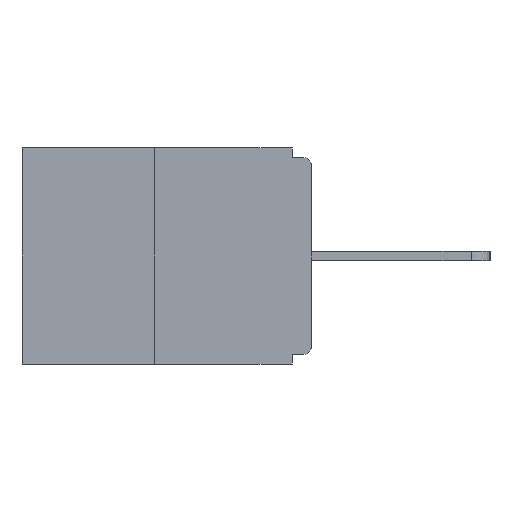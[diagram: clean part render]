
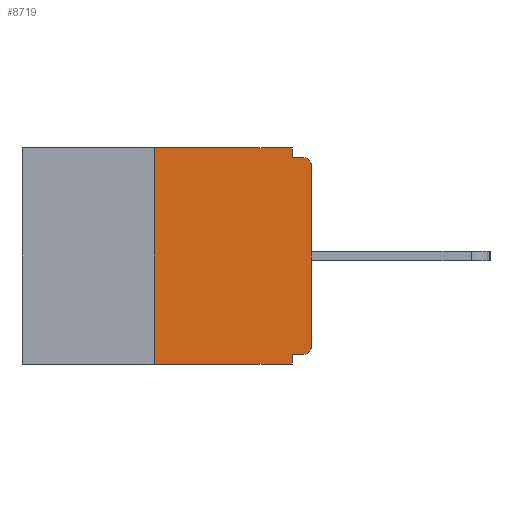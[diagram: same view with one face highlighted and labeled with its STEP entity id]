
A CAD part, left-side view. The second image highlights one B-rep face of the part: STEP entity #8719.
In plain terms, the highlighted planar face has unit normal (-1, 0, 0).
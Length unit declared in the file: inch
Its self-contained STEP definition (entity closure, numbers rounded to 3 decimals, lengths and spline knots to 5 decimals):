
#188 = CARTESIAN_POINT ( 'NONE',  ( 0., 0.031, 0. ) ) ;
#361 = ORIENTED_EDGE ( 'NONE', *, *, #2135, .F. ) ;
#524 = LINE ( 'NONE', #4697, #8600 ) ;
#560 = CARTESIAN_POINT ( 'NONE',  ( 0., 0.25, 0. ) ) ;
#567 = ORIENTED_EDGE ( 'NONE', *, *, #5342, .F. ) ;
#771 = DIRECTION ( 'NONE',  ( 1., 0., 0. ) ) ;
#990 = DIRECTION ( 'NONE',  ( 0., 0., -1. ) ) ;
#1240 = LINE ( 'NONE', #10853, #4641 ) ;
#1313 = CARTESIAN_POINT ( 'NONE',  ( 0., 0., -0.328 ) ) ;
#1405 = AXIS2_PLACEMENT_3D ( 'NONE', #8255, #771, #9372 ) ;
#1598 = CIRCLE ( 'NONE', #12815, 0.015 ) ;
#1734 = EDGE_LOOP ( 'NONE', ( #7127, #5893, #7165, #567, #10766, #7351, #2995, #6404, #7505, #361 ) ) ;
#1804 = DIRECTION ( 'NONE',  ( 0., -1., 0. ) ) ;
#1980 = CARTESIAN_POINT ( 'NONE',  ( 0., 0.015, -0.015 ) ) ;
#2005 = FACE_OUTER_BOUND ( 'NONE', #1734, .T. ) ;
#2135 = EDGE_CURVE ( 'NONE', #13423, #8696, #4157, .T. ) ;
#2299 = VECTOR ( 'NONE', #1804, 39.37008 ) ;
#2954 = CARTESIAN_POINT ( 'NONE',  ( 0., 0.031, -0.328 ) ) ;
#2995 = ORIENTED_EDGE ( 'NONE', *, *, #7608, .T. ) ;
#3349 = VERTEX_POINT ( 'NONE', #7394 ) ;
#3566 = DIRECTION ( 'NONE',  ( 0., 1., 0. ) ) ;
#3804 = VECTOR ( 'NONE', #9778, 39.37008 ) ;
#3986 = CARTESIAN_POINT ( 'NONE',  ( 0., 0., -0.015 ) ) ;
#4157 = LINE ( 'NONE', #188, #4753 ) ;
#4296 = DIRECTION ( 'NONE',  ( 0., 0., 1. ) ) ;
#4641 = VECTOR ( 'NONE', #4296, 39.37008 ) ;
#4697 = CARTESIAN_POINT ( 'NONE',  ( 0., 0.46, -0.343 ) ) ;
#4753 = VECTOR ( 'NONE', #5257, 39.37008 ) ;
#4831 = CARTESIAN_POINT ( 'NONE',  ( 0., 0.031, 0. ) ) ;
#5257 = DIRECTION ( 'NONE',  ( 0., 0., -1. ) ) ;
#5342 = EDGE_CURVE ( 'NONE', #7071, #12748, #8388, .T. ) ;
#5519 = EDGE_CURVE ( 'NONE', #10496, #13423, #8584, .T. ) ;
#5863 = VERTEX_POINT ( 'NONE', #7185 ) ;
#5893 = ORIENTED_EDGE ( 'NONE', *, *, #10314, .F. ) ;
#6404 = ORIENTED_EDGE ( 'NONE', *, *, #6942, .T. ) ;
#6863 = LINE ( 'NONE', #1313, #9118 ) ;
#6876 = DIRECTION ( 'NONE',  ( 0., 0., -1. ) ) ;
#6942 = EDGE_CURVE ( 'NONE', #3349, #12597, #1598, .T. ) ;
#7071 = VERTEX_POINT ( 'NONE', #2954 ) ;
#7127 = ORIENTED_EDGE ( 'NONE', *, *, #5519, .F. ) ;
#7131 = CARTESIAN_POINT ( 'NONE',  ( 0., 0.25, 0. ) ) ;
#7165 = ORIENTED_EDGE ( 'NONE', *, *, #7809, .T. ) ;
#7185 = CARTESIAN_POINT ( 'NONE',  ( 0., 0.015, -0.328 ) ) ;
#7351 = ORIENTED_EDGE ( 'NONE', *, *, #13072, .T. ) ;
#7394 = CARTESIAN_POINT ( 'NONE',  ( 0., 0., -0.03 ) ) ;
#7416 = VERTEX_POINT ( 'NONE', #13518 ) ;
#7505 = ORIENTED_EDGE ( 'NONE', *, *, #13149, .F. ) ;
#7608 = EDGE_CURVE ( 'NONE', #11166, #3349, #1240, .T. ) ;
#7755 = AXIS2_PLACEMENT_3D ( 'NONE', #8949, #9095, #6876 ) ;
#7809 = EDGE_CURVE ( 'NONE', #7416, #12748, #524, .T. ) ;
#8102 = PLANE ( 'NONE',  #1405 ) ;
#8255 = CARTESIAN_POINT ( 'NONE',  ( 0., 0.46, 0. ) ) ;
#8388 = LINE ( 'NONE', #10546, #11446 ) ;
#8560 = CARTESIAN_POINT ( 'NONE',  ( 0., 0., -0.313 ) ) ;
#8584 = LINE ( 'NONE', #12832, #9665 ) ;
#8600 = VECTOR ( 'NONE', #8921, 39.37008 ) ;
#8696 = VERTEX_POINT ( 'NONE', #13598 ) ;
#8719 = ADVANCED_FACE ( 'NONE', ( #2005 ), #8102, .F. ) ;
#8921 = DIRECTION ( 'NONE',  ( 0., -1., 0. ) ) ;
#8949 = CARTESIAN_POINT ( 'NONE',  ( 0., 0.015, -0.313 ) ) ;
#9095 = DIRECTION ( 'NONE',  ( -1., 0., 0. ) ) ;
#9118 = VECTOR ( 'NONE', #3566, 39.37008 ) ;
#9372 = DIRECTION ( 'NONE',  ( 0., 0., -1. ) ) ;
#9665 = VECTOR ( 'NONE', #10749, 39.37008 ) ;
#9778 = DIRECTION ( 'NONE',  ( 0., 0., 1. ) ) ;
#10314 = EDGE_CURVE ( 'NONE', #7416, #10496, #12143, .T. ) ;
#10496 = VERTEX_POINT ( 'NONE', #7131 ) ;
#10546 = CARTESIAN_POINT ( 'NONE',  ( 0., 0.031, -0.343 ) ) ;
#10649 = CIRCLE ( 'NONE', #7755, 0.015 ) ;
#10719 = CARTESIAN_POINT ( 'NONE',  ( 0., 0.031, -0.343 ) ) ;
#10749 = DIRECTION ( 'NONE',  ( 0., -1., 0. ) ) ;
#10766 = ORIENTED_EDGE ( 'NONE', *, *, #12026, .F. ) ;
#10853 = CARTESIAN_POINT ( 'NONE',  ( 0., 0., 0. ) ) ;
#10906 = CARTESIAN_POINT ( 'NONE',  ( 0., 0.015, -0.03 ) ) ;
#11166 = VERTEX_POINT ( 'NONE', #8560 ) ;
#11436 = DIRECTION ( 'NONE',  ( -1., 0., 0. ) ) ;
#11446 = VECTOR ( 'NONE', #990, 39.37008 ) ;
#12026 = EDGE_CURVE ( 'NONE', #5863, #7071, #6863, .T. ) ;
#12143 = LINE ( 'NONE', #560, #3804 ) ;
#12351 = LINE ( 'NONE', #3986, #2299 ) ;
#12550 = DIRECTION ( 'NONE',  ( 0., 0., -1. ) ) ;
#12597 = VERTEX_POINT ( 'NONE', #1980 ) ;
#12748 = VERTEX_POINT ( 'NONE', #10719 ) ;
#12815 = AXIS2_PLACEMENT_3D ( 'NONE', #10906, #11436, #12550 ) ;
#12832 = CARTESIAN_POINT ( 'NONE',  ( 0., 0.46, 0. ) ) ;
#13072 = EDGE_CURVE ( 'NONE', #5863, #11166, #10649, .T. ) ;
#13149 = EDGE_CURVE ( 'NONE', #8696, #12597, #12351, .T. ) ;
#13423 = VERTEX_POINT ( 'NONE', #4831 ) ;
#13518 = CARTESIAN_POINT ( 'NONE',  ( 0., 0.25, -0.343 ) ) ;
#13598 = CARTESIAN_POINT ( 'NONE',  ( 0., 0.031, -0.015 ) ) ;
